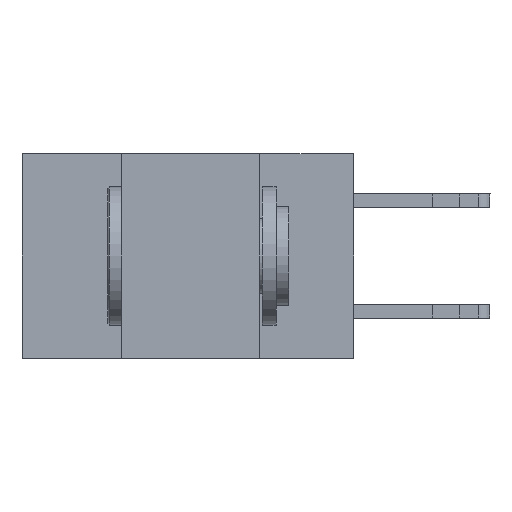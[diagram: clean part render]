
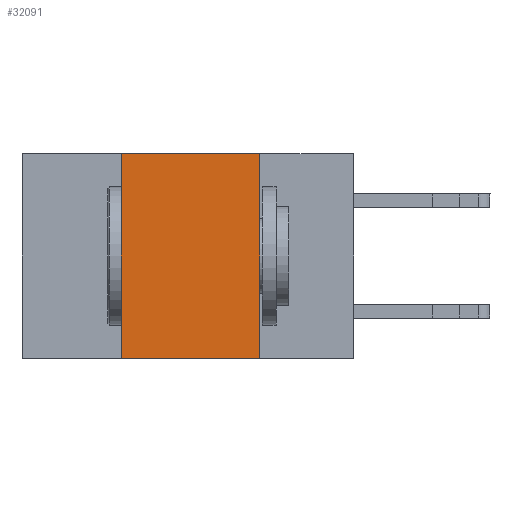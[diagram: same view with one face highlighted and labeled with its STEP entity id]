
A CAD part, left-side view. The second image highlights one B-rep face of the part: STEP entity #32091.
In plain terms, the highlighted planar face has unit normal (-1, 0, 0).
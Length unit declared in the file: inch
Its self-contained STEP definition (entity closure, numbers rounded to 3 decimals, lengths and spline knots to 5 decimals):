
#42 = DIRECTION ( 'NONE',  ( 0., 0., 1. ) ) ;
#2131 = CARTESIAN_POINT ( 'NONE',  ( 0., 0.17, -0.37 ) ) ;
#3662 = LINE ( 'NONE', #11782, #27275 ) ;
#4306 = CARTESIAN_POINT ( 'NONE',  ( 0., 0.17, 0. ) ) ;
#5015 = CARTESIAN_POINT ( 'NONE',  ( 0., 0.17, 0. ) ) ;
#5599 = EDGE_LOOP ( 'NONE', ( #26518, #34411, #13990, #24219 ) ) ;
#5660 = PLANE ( 'NONE',  #29971 ) ;
#5952 = VERTEX_POINT ( 'NONE', #9488 ) ;
#8903 = CARTESIAN_POINT ( 'NONE',  ( 0., 0.6, 0. ) ) ;
#9488 = CARTESIAN_POINT ( 'NONE',  ( 0., 0.42, -0.37 ) ) ;
#11631 = DIRECTION ( 'NONE',  ( 1., 0., 0. ) ) ;
#11782 = CARTESIAN_POINT ( 'NONE',  ( 0., 0.42, 0. ) ) ;
#12519 = EDGE_CURVE ( 'NONE', #30076, #19010, #37290, .T. ) ;
#13990 = ORIENTED_EDGE ( 'NONE', *, *, #37268, .F. ) ;
#14131 = CARTESIAN_POINT ( 'NONE',  ( 0., 0.42, 0. ) ) ;
#14480 = VECTOR ( 'NONE', #28297, 39.37008 ) ;
#15011 = DIRECTION ( 'NONE',  ( 0., -1., 0. ) ) ;
#17478 = CARTESIAN_POINT ( 'NONE',  ( 0., 0.6, 0. ) ) ;
#18393 = VECTOR ( 'NONE', #15011, 39.37008 ) ;
#19010 = VERTEX_POINT ( 'NONE', #4306 ) ;
#23244 = DIRECTION ( 'NONE',  ( 0., 0., -1. ) ) ;
#24219 = ORIENTED_EDGE ( 'NONE', *, *, #36112, .T. ) ;
#26518 = ORIENTED_EDGE ( 'NONE', *, *, #32246, .F. ) ;
#27275 = VECTOR ( 'NONE', #42, 39.37008 ) ;
#28297 = DIRECTION ( 'NONE',  ( 0., -1., 0. ) ) ;
#28802 = CARTESIAN_POINT ( 'NONE',  ( 0., 0.6, -0.37 ) ) ;
#29180 = DIRECTION ( 'NONE',  ( 0., 0., -1. ) ) ;
#29971 = AXIS2_PLACEMENT_3D ( 'NONE', #17478, #11631, #23244 ) ;
#30076 = VERTEX_POINT ( 'NONE', #14131 ) ;
#31094 = LINE ( 'NONE', #28802, #14480 ) ;
#31464 = VERTEX_POINT ( 'NONE', #2131 ) ;
#32091 = ADVANCED_FACE ( 'NONE', ( #33700 ), #5660, .F. ) ;
#32246 = EDGE_CURVE ( 'NONE', #19010, #31464, #36490, .T. ) ;
#33700 = FACE_OUTER_BOUND ( 'NONE', #5599, .T. ) ;
#34232 = VECTOR ( 'NONE', #29180, 39.37008 ) ;
#34411 = ORIENTED_EDGE ( 'NONE', *, *, #12519, .F. ) ;
#36112 = EDGE_CURVE ( 'NONE', #5952, #31464, #31094, .T. ) ;
#36490 = LINE ( 'NONE', #5015, #34232 ) ;
#37268 = EDGE_CURVE ( 'NONE', #5952, #30076, #3662, .T. ) ;
#37290 = LINE ( 'NONE', #8903, #18393 ) ;
